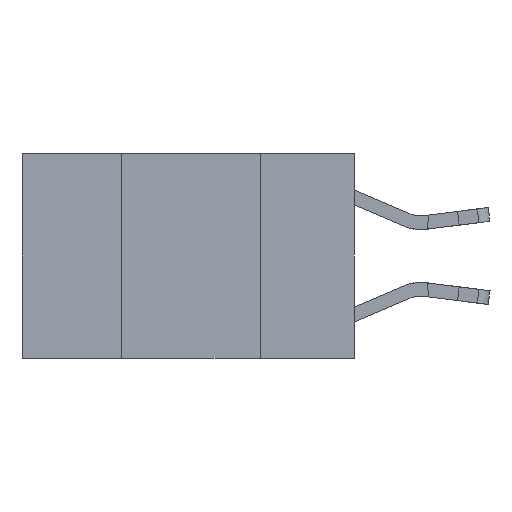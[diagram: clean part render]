
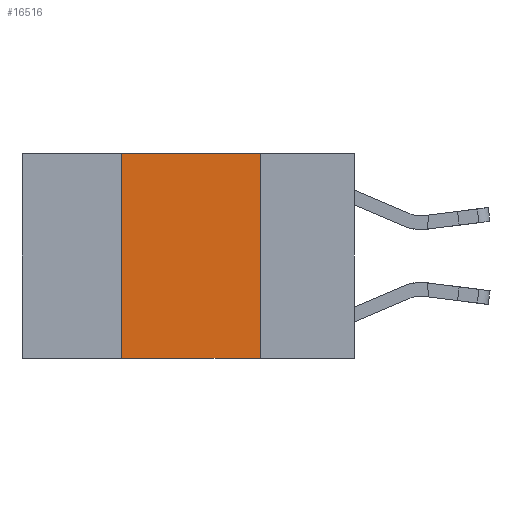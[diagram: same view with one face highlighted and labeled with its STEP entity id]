
A CAD part, left-side view. The second image highlights one B-rep face of the part: STEP entity #16516.
In plain terms, the highlighted planar face has unit normal (-1, 0, 0).
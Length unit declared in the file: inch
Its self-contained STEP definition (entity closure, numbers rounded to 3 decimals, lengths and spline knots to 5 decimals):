
#978 = EDGE_CURVE ( 'NONE', #16177, #7309, #9655, .T. ) ;
#1485 = VECTOR ( 'NONE', #15126, 39.37008 ) ;
#3057 = VERTEX_POINT ( 'NONE', #12396 ) ;
#3889 = CARTESIAN_POINT ( 'NONE',  ( 0., 0.17, 0. ) ) ;
#4157 = ORIENTED_EDGE ( 'NONE', *, *, #14745, .F. ) ;
#4393 = CARTESIAN_POINT ( 'NONE',  ( 0., 0.42, 0. ) ) ;
#4604 = LINE ( 'NONE', #9148, #12171 ) ;
#4725 = EDGE_CURVE ( 'NONE', #19420, #16177, #10965, .T. ) ;
#5380 = DIRECTION ( 'NONE',  ( 1., 0., 0. ) ) ;
#6480 = VECTOR ( 'NONE', #14860, 39.37008 ) ;
#7309 = VERTEX_POINT ( 'NONE', #16406 ) ;
#7366 = CARTESIAN_POINT ( 'NONE',  ( 0., 0.6, 0. ) ) ;
#8285 = AXIS2_PLACEMENT_3D ( 'NONE', #17358, #5380, #15923 ) ;
#8665 = ORIENTED_EDGE ( 'NONE', *, *, #4725, .F. ) ;
#8700 = VECTOR ( 'NONE', #11951, 39.37008 ) ;
#9083 = CARTESIAN_POINT ( 'NONE',  ( 0., 0.6, -0.37 ) ) ;
#9148 = CARTESIAN_POINT ( 'NONE',  ( 0., 0.42, 0. ) ) ;
#9363 = EDGE_LOOP ( 'NONE', ( #17127, #8665, #4157, #15722 ) ) ;
#9655 = LINE ( 'NONE', #3889, #8700 ) ;
#10645 = DIRECTION ( 'NONE',  ( 0., 0., 1. ) ) ;
#10965 = LINE ( 'NONE', #7366, #6480 ) ;
#11615 = FACE_OUTER_BOUND ( 'NONE', #9363, .T. ) ;
#11951 = DIRECTION ( 'NONE',  ( 0., 0., -1. ) ) ;
#12125 = CARTESIAN_POINT ( 'NONE',  ( 0., 0.17, 0. ) ) ;
#12171 = VECTOR ( 'NONE', #10645, 39.37008 ) ;
#12396 = CARTESIAN_POINT ( 'NONE',  ( 0., 0.42, -0.37 ) ) ;
#14745 = EDGE_CURVE ( 'NONE', #3057, #19420, #4604, .T. ) ;
#14860 = DIRECTION ( 'NONE',  ( 0., -1., 0. ) ) ;
#15126 = DIRECTION ( 'NONE',  ( 0., -1., 0. ) ) ;
#15722 = ORIENTED_EDGE ( 'NONE', *, *, #16849, .T. ) ;
#15923 = DIRECTION ( 'NONE',  ( 0., 0., -1. ) ) ;
#16177 = VERTEX_POINT ( 'NONE', #12125 ) ;
#16406 = CARTESIAN_POINT ( 'NONE',  ( 0., 0.17, -0.37 ) ) ;
#16516 = ADVANCED_FACE ( 'NONE', ( #11615 ), #18869, .F. ) ;
#16849 = EDGE_CURVE ( 'NONE', #3057, #7309, #18065, .T. ) ;
#17127 = ORIENTED_EDGE ( 'NONE', *, *, #978, .F. ) ;
#17358 = CARTESIAN_POINT ( 'NONE',  ( 0., 0.6, 0. ) ) ;
#18065 = LINE ( 'NONE', #9083, #1485 ) ;
#18869 = PLANE ( 'NONE',  #8285 ) ;
#19420 = VERTEX_POINT ( 'NONE', #4393 ) ;
